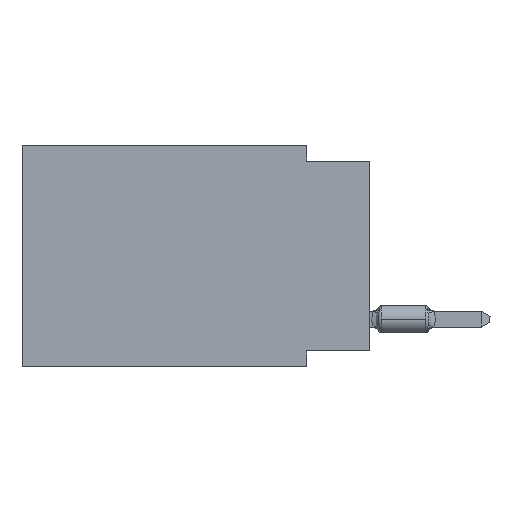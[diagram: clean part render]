
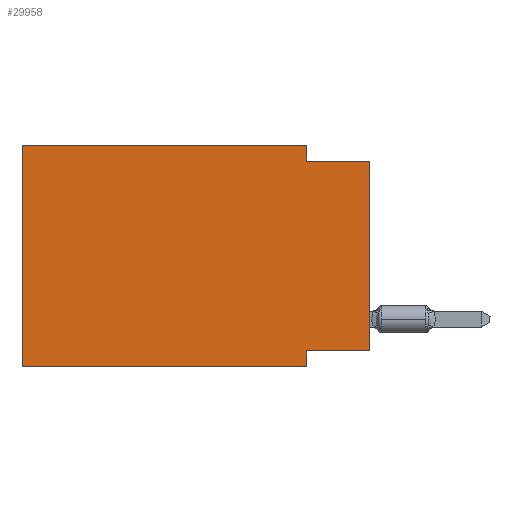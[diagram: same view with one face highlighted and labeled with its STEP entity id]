
A CAD part, left-side view. The second image highlights one B-rep face of the part: STEP entity #29958.
In plain terms, the highlighted planar face has unit normal (-1, 0, 0).
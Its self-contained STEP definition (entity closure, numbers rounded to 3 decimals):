
#656 = LINE ( 'NONE', #34135, #12016 ) ;
#3414 = VECTOR ( 'NONE', #70332, 1000. ) ;
#4103 = CARTESIAN_POINT ( 'NONE',  ( 0., 2.54, -8.89 ) ) ;
#6813 = PLANE ( 'NONE',  #80913 ) ;
#8891 = DIRECTION ( 'NONE',  ( 0., -1., 0. ) ) ;
#10472 = VECTOR ( 'NONE', #64293, 1000. ) ;
#12016 = VECTOR ( 'NONE', #66304, 1000. ) ;
#12468 = FACE_OUTER_BOUND ( 'NONE', #21139, .T. ) ;
#14453 = EDGE_CURVE ( 'NONE', #33796, #58169, #44325, .T. ) ;
#15462 = ORIENTED_EDGE ( 'NONE', *, *, #14453, .F. ) ;
#15634 = CARTESIAN_POINT ( 'NONE',  ( 0., 13.97, 0. ) ) ;
#16922 = CARTESIAN_POINT ( 'NONE',  ( 0., 13.97, 0. ) ) ;
#18258 = LINE ( 'NONE', #39133, #83239 ) ;
#20949 = CARTESIAN_POINT ( 'NONE',  ( 0., 0., -8.255 ) ) ;
#21139 = EDGE_LOOP ( 'NONE', ( #49759, #78627, #77275, #74153, #21908, #57085, #15462, #68368 ) ) ;
#21908 = ORIENTED_EDGE ( 'NONE', *, *, #43483, .F. ) ;
#22724 = VECTOR ( 'NONE', #55799, 1000. ) ;
#24914 = DIRECTION ( 'NONE',  ( 0., -1., 0. ) ) ;
#28039 = VECTOR ( 'NONE', #24914, 1000. ) ;
#28514 = EDGE_CURVE ( 'NONE', #51424, #70267, #71858, .T. ) ;
#29958 = ADVANCED_FACE ( 'NONE', ( #12468 ), #6813, .F. ) ;
#33757 = CARTESIAN_POINT ( 'NONE',  ( 0., 13.97, 0. ) ) ;
#33796 = VERTEX_POINT ( 'NONE', #60812 ) ;
#34135 = CARTESIAN_POINT ( 'NONE',  ( 0., 13.97, -8.89 ) ) ;
#34971 = LINE ( 'NONE', #81070, #48238 ) ;
#35645 = DIRECTION ( 'NONE',  ( 0., 0., 1. ) ) ;
#39133 = CARTESIAN_POINT ( 'NONE',  ( 0., 2.54, 0. ) ) ;
#42099 = EDGE_CURVE ( 'NONE', #75107, #51424, #18258, .T. ) ;
#43483 = EDGE_CURVE ( 'NONE', #72854, #76164, #68245, .T. ) ;
#44040 = CARTESIAN_POINT ( 'NONE',  ( 0., 0., -8.255 ) ) ;
#44325 = LINE ( 'NONE', #50006, #10472 ) ;
#45343 = CARTESIAN_POINT ( 'NONE',  ( 0., 0., -0.635 ) ) ;
#45740 = CARTESIAN_POINT ( 'NONE',  ( 0., 2.54, -0.635 ) ) ;
#46802 = DIRECTION ( 'NONE',  ( 1., 0., 0. ) ) ;
#48238 = VECTOR ( 'NONE', #8891, 1000. ) ;
#49759 = ORIENTED_EDGE ( 'NONE', *, *, #52140, .T. ) ;
#50006 = CARTESIAN_POINT ( 'NONE',  ( 0., 2.54, -8.89 ) ) ;
#51234 = EDGE_CURVE ( 'NONE', #65816, #33796, #82328, .T. ) ;
#51424 = VERTEX_POINT ( 'NONE', #45740 ) ;
#52140 = EDGE_CURVE ( 'NONE', #65816, #70267, #85609, .T. ) ;
#55471 = EDGE_CURVE ( 'NONE', #76164, #75107, #34971, .T. ) ;
#55799 = DIRECTION ( 'NONE',  ( 0., 1., 0. ) ) ;
#56700 = CARTESIAN_POINT ( 'NONE',  ( 0., 0., -0.635 ) ) ;
#56759 = EDGE_CURVE ( 'NONE', #72854, #58169, #656, .T. ) ;
#57085 = ORIENTED_EDGE ( 'NONE', *, *, #56759, .T. ) ;
#58169 = VERTEX_POINT ( 'NONE', #4103 ) ;
#60812 = CARTESIAN_POINT ( 'NONE',  ( 0., 2.54, -8.255 ) ) ;
#63502 = CARTESIAN_POINT ( 'NONE',  ( 0., 2.54, 0. ) ) ;
#64293 = DIRECTION ( 'NONE',  ( 0., 0., -1. ) ) ;
#65816 = VERTEX_POINT ( 'NONE', #20949 ) ;
#66304 = DIRECTION ( 'NONE',  ( 0., -1., 0. ) ) ;
#66358 = DIRECTION ( 'NONE',  ( 0., 0., -1. ) ) ;
#66460 = CARTESIAN_POINT ( 'NONE',  ( 0., 0., 0. ) ) ;
#68245 = LINE ( 'NONE', #15634, #75058 ) ;
#68368 = ORIENTED_EDGE ( 'NONE', *, *, #51234, .F. ) ;
#70267 = VERTEX_POINT ( 'NONE', #56700 ) ;
#70332 = DIRECTION ( 'NONE',  ( 0., 0., 1. ) ) ;
#71299 = DIRECTION ( 'NONE',  ( 0., 0., -1. ) ) ;
#71858 = LINE ( 'NONE', #45343, #28039 ) ;
#72854 = VERTEX_POINT ( 'NONE', #72992 ) ;
#72992 = CARTESIAN_POINT ( 'NONE',  ( 0., 13.97, -8.89 ) ) ;
#74153 = ORIENTED_EDGE ( 'NONE', *, *, #55471, .F. ) ;
#75058 = VECTOR ( 'NONE', #35645, 1000. ) ;
#75107 = VERTEX_POINT ( 'NONE', #63502 ) ;
#76164 = VERTEX_POINT ( 'NONE', #16922 ) ;
#77275 = ORIENTED_EDGE ( 'NONE', *, *, #42099, .F. ) ;
#78627 = ORIENTED_EDGE ( 'NONE', *, *, #28514, .F. ) ;
#80913 = AXIS2_PLACEMENT_3D ( 'NONE', #33757, #46802, #66358 ) ;
#81070 = CARTESIAN_POINT ( 'NONE',  ( 0., 13.97, 0. ) ) ;
#82328 = LINE ( 'NONE', #44040, #22724 ) ;
#83239 = VECTOR ( 'NONE', #71299, 1000. ) ;
#85609 = LINE ( 'NONE', #66460, #3414 ) ;
